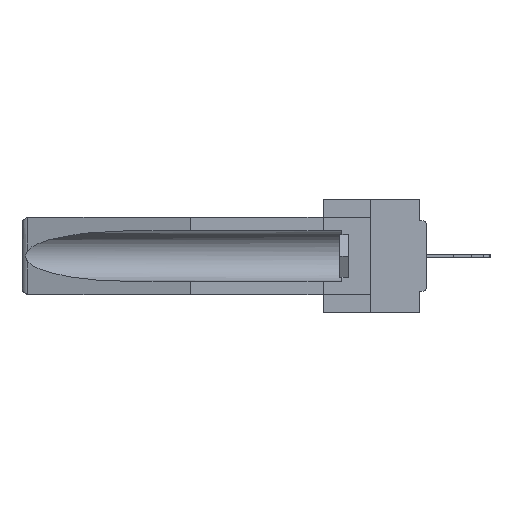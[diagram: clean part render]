
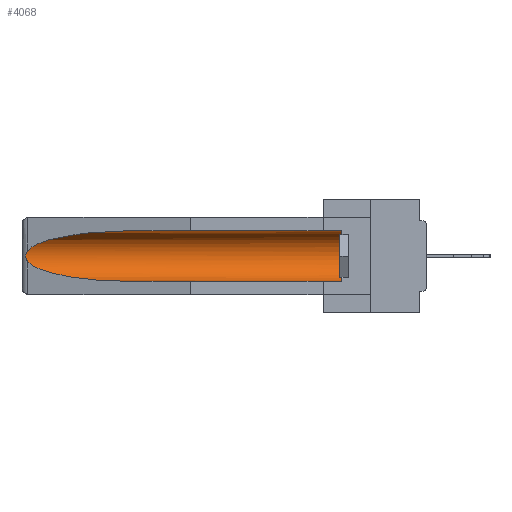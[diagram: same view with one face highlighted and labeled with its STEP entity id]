
A CAD part, left-side view. The second image highlights one B-rep face of the part: STEP entity #4068.
In plain terms, the highlighted cylindrical face has radius 2.857 mm (diameter 5.715 mm), a partial arc.
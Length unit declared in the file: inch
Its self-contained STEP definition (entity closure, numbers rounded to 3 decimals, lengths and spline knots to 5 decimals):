
#1688 =( BOUNDED_CURVE ( )  B_SPLINE_CURVE ( 3, ( #7435, #19082, #34372, #11063 ),
 .UNSPECIFIED., .F., .F. ) 
 B_SPLINE_CURVE_WITH_KNOTS ( ( 4, 4 ),
 ( 0.1948, 1.5708 ),
 .UNSPECIFIED. ) 
 CURVE ( )  GEOMETRIC_REPRESENTATION_ITEM ( )  RATIONAL_B_SPLINE_CURVE ( ( 1., 0.848, 0.848, 1. ) ) 
 REPRESENTATION_ITEM ( '' )  );
#2206 = DIRECTION ( 'NONE',  ( 0., -1., 0. ) ) ;
#2679 = ORIENTED_EDGE ( 'NONE', *, *, #4332, .T. ) ;
#3813 = CARTESIAN_POINT ( 'NONE',  ( 0.26654, 1.53092, -0.15636 ) ) ;
#4068 = ADVANCED_FACE ( 'NONE', ( #27826 ), #30504, .F. ) ;
#4332 = EDGE_CURVE ( 'NONE', #35765, #7239, #15123, .T. ) ;
#5673 = ORIENTED_EDGE ( 'NONE', *, *, #34121, .F. ) ;
#5908 = CARTESIAN_POINT ( 'NONE',  ( 0.155, -0.30754, -0.284 ) ) ;
#6521 = VECTOR ( 'NONE', #32701, 39.37008 ) ;
#6611 = CIRCLE ( 'NONE', #37127, 0.1125 ) ;
#6690 = CARTESIAN_POINT ( 'NONE',  ( 0.26537, 1.52718, -0.14972 ) ) ;
#7030 = EDGE_CURVE ( 'NONE', #19950, #35765, #6611, .T. ) ;
#7239 = VERTEX_POINT ( 'NONE', #23211 ) ;
#7435 = CARTESIAN_POINT ( 'NONE',  ( 0.26537, 1.52718, -0.19328 ) ) ;
#7553 = CARTESIAN_POINT ( 'NONE',  ( 0.155, -0.30754, -0.1715 ) ) ;
#7718 = CARTESIAN_POINT ( 'NONE',  ( 0.155, 1.07973, -0.059 ) ) ;
#8035 = ORIENTED_EDGE ( 'NONE', *, *, #15965, .T. ) ;
#9156 = LINE ( 'NONE', #5908, #15486 ) ;
#9268 =( BOUNDED_CURVE ( )  B_SPLINE_CURVE ( 3, ( #7718, #10227, #31427, #19184 ),
 .UNSPECIFIED., .F., .F. ) 
 B_SPLINE_CURVE_WITH_KNOTS ( ( 4, 4 ),
 ( 4.71239, 6.08839 ),
 .UNSPECIFIED. ) 
 CURVE ( )  GEOMETRIC_REPRESENTATION_ITEM ( )  RATIONAL_B_SPLINE_CURVE ( ( 1., 0.848, 0.848, 1. ) ) 
 REPRESENTATION_ITEM ( '' )  );
#10227 = CARTESIAN_POINT ( 'NONE',  ( 0.21114, 1.30732, -0.059 ) ) ;
#10700 = CARTESIAN_POINT ( 'NONE',  ( 0.155, 1.07973, -0.284 ) ) ;
#10762 = CARTESIAN_POINT ( 'NONE',  ( 0.26537, 1.52718, -0.19328 ) ) ;
#11048 = EDGE_LOOP ( 'NONE', ( #20382, #16358, #8035, #5673, #29347, #2679 ) ) ;
#11063 = CARTESIAN_POINT ( 'NONE',  ( 0.155, 1.07973, -0.284 ) ) ;
#11924 = VERTEX_POINT ( 'NONE', #10700 ) ;
#12427 = CARTESIAN_POINT ( 'NONE',  ( 0.26597, 1.52961, -0.15275 ) ) ;
#13856 = DIRECTION ( 'NONE',  ( 0., 0., 1. ) ) ;
#15123 = LINE ( 'NONE', #33282, #6521 ) ;
#15486 = VECTOR ( 'NONE', #17570, 39.37008 ) ;
#15965 = EDGE_CURVE ( 'NONE', #24947, #11924, #1688, .T. ) ;
#16358 = ORIENTED_EDGE ( 'NONE', *, *, #17075, .T. ) ;
#17075 = EDGE_CURVE ( 'NONE', #35806, #24947, #20748, .T. ) ;
#17570 = DIRECTION ( 'NONE',  ( 0., 1., 0. ) ) ;
#18718 = CARTESIAN_POINT ( 'NONE',  ( 0.26537, 1.52718, -0.19328 ) ) ;
#19082 = CARTESIAN_POINT ( 'NONE',  ( 0.25451, 1.48313, -0.24835 ) ) ;
#19184 = CARTESIAN_POINT ( 'NONE',  ( 0.26537, 1.52718, -0.14972 ) ) ;
#19950 = VERTEX_POINT ( 'NONE', #36404 ) ;
#20382 = ORIENTED_EDGE ( 'NONE', *, *, #29717, .T. ) ;
#20748 = B_SPLINE_CURVE_WITH_KNOTS ( 'NONE', 3,
 ( #6690, #12427, #3813, #30394, #24067, #35741, #27333, #30212, #27717, #18718 ),
 .UNSPECIFIED., .F., .F.,
 ( 4, 2, 2, 2, 4 ),
 ( 0., 0.00029, 0.00058, 0.00087, 0.00117 ),
 .UNSPECIFIED. ) ;
#21361 = CARTESIAN_POINT ( 'NONE',  ( 0.26537, 1.52718, -0.14972 ) ) ;
#21508 = DIRECTION ( 'NONE',  ( 0., 1., 0. ) ) ;
#23211 = CARTESIAN_POINT ( 'NONE',  ( 0.155, 1.07973, -0.059 ) ) ;
#24067 = CARTESIAN_POINT ( 'NONE',  ( 0.2675, 1.53308, -0.16763 ) ) ;
#24947 = VERTEX_POINT ( 'NONE', #10762 ) ;
#27333 = CARTESIAN_POINT ( 'NONE',  ( 0.2673, 1.53269, -0.17917 ) ) ;
#27717 = CARTESIAN_POINT ( 'NONE',  ( 0.26597, 1.5296, -0.19026 ) ) ;
#27826 = FACE_OUTER_BOUND ( 'NONE', #11048, .T. ) ;
#29347 = ORIENTED_EDGE ( 'NONE', *, *, #7030, .T. ) ;
#29669 = AXIS2_PLACEMENT_3D ( 'NONE', #7553, #21508, #30887 ) ;
#29717 = EDGE_CURVE ( 'NONE', #7239, #35806, #9268, .T. ) ;
#30212 = CARTESIAN_POINT ( 'NONE',  ( 0.26655, 1.53094, -0.18657 ) ) ;
#30394 = CARTESIAN_POINT ( 'NONE',  ( 0.2673, 1.5327, -0.16383 ) ) ;
#30504 = CYLINDRICAL_SURFACE ( 'NONE', #29669, 0.1125 ) ;
#30887 = DIRECTION ( 'NONE',  ( 0., 0., 1. ) ) ;
#31427 = CARTESIAN_POINT ( 'NONE',  ( 0.25451, 1.48313, -0.09465 ) ) ;
#32701 = DIRECTION ( 'NONE',  ( 0., 1., 0. ) ) ;
#33282 = CARTESIAN_POINT ( 'NONE',  ( 0.155, -0.30754, -0.059 ) ) ;
#33929 = CARTESIAN_POINT ( 'NONE',  ( 0.155, 0.126, -0.059 ) ) ;
#33941 = CARTESIAN_POINT ( 'NONE',  ( 0.155, 0.126, -0.1715 ) ) ;
#34121 = EDGE_CURVE ( 'NONE', #19950, #11924, #9156, .T. ) ;
#34372 = CARTESIAN_POINT ( 'NONE',  ( 0.21114, 1.30732, -0.284 ) ) ;
#35741 = CARTESIAN_POINT ( 'NONE',  ( 0.2675, 1.53308, -0.17534 ) ) ;
#35765 = VERTEX_POINT ( 'NONE', #33929 ) ;
#35806 = VERTEX_POINT ( 'NONE', #21361 ) ;
#36404 = CARTESIAN_POINT ( 'NONE',  ( 0.155, 0.126, -0.284 ) ) ;
#37127 = AXIS2_PLACEMENT_3D ( 'NONE', #33941, #2206, #13856 ) ;
